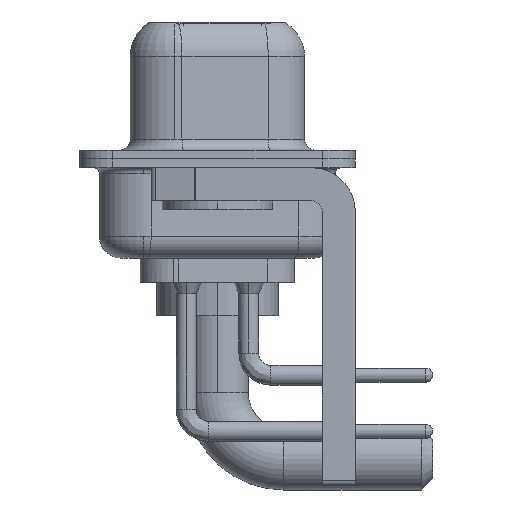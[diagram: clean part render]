
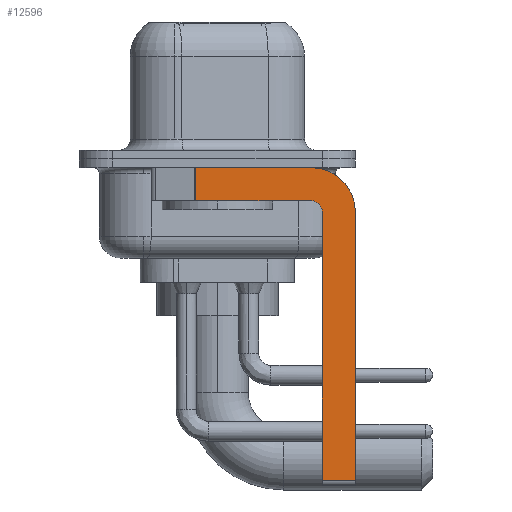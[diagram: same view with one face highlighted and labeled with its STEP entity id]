
A CAD part, left-side view. The second image highlights one B-rep face of the part: STEP entity #12596.
In plain terms, the highlighted planar face has unit normal (-1, 0, 0).
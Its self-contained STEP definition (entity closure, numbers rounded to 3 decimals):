
#85 = ORIENTED_EDGE ( 'NONE', *, *, #14228, .F. ) ;
#259 = LINE ( 'NONE', #1392, #5265 ) ;
#366 = VERTEX_POINT ( 'NONE', #14176 ) ;
#626 = DIRECTION ( 'NONE',  ( 0., 0., -1. ) ) ;
#1088 = LINE ( 'NONE', #5089, #1661 ) ;
#1392 = CARTESIAN_POINT ( 'NONE',  ( -2.9, -6.25, -2.4 ) ) ;
#1661 = VECTOR ( 'NONE', #9052, 1000. ) ;
#1817 = CARTESIAN_POINT ( 'NONE',  ( -2.9, 0.978, -1.9 ) ) ;
#1922 = FACE_OUTER_BOUND ( 'NONE', #5949, .T. ) ;
#2211 = VERTEX_POINT ( 'NONE', #9523 ) ;
#2514 = VECTOR ( 'NONE', #17074, 1000. ) ;
#2653 = VECTOR ( 'NONE', #3198, 1000. ) ;
#2788 = DIRECTION ( 'NONE',  ( 0., 0., -1. ) ) ;
#2790 = CIRCLE ( 'NONE', #15186, 0.5 ) ;
#3198 = DIRECTION ( 'NONE',  ( 0., 0., 1. ) ) ;
#3204 = CARTESIAN_POINT ( 'NONE',  ( -2.9, -4.25, -2.4 ) ) ;
#3291 = DIRECTION ( 'NONE',  ( 0., -1., 0. ) ) ;
#3436 = AXIS2_PLACEMENT_3D ( 'NONE', #14606, #17026, #2788 ) ;
#4014 = ORIENTED_EDGE ( 'NONE', *, *, #5808, .F. ) ;
#4592 = CARTESIAN_POINT ( 'NONE',  ( -2.9, 3., -0.4 ) ) ;
#4657 = VECTOR ( 'NONE', #3291, 1000. ) ;
#4873 = DIRECTION ( 'NONE',  ( 0., -1., 0. ) ) ;
#4947 = EDGE_CURVE ( 'NONE', #15247, #366, #14741, .T. ) ;
#5089 = CARTESIAN_POINT ( 'NONE',  ( -2.9, -4.25, -1.9 ) ) ;
#5265 = VECTOR ( 'NONE', #8153, 1000. ) ;
#5554 = ORIENTED_EDGE ( 'NONE', *, *, #7724, .F. ) ;
#5808 = EDGE_CURVE ( 'NONE', #10435, #2211, #11835, .T. ) ;
#5831 = VERTEX_POINT ( 'NONE', #13481 ) ;
#5949 = EDGE_LOOP ( 'NONE', ( #5554, #12577, #14090, #11803, #4014, #13817, #85, #15540 ) ) ;
#5972 = CARTESIAN_POINT ( 'NONE',  ( -2.9, -4.25, -2.4 ) ) ;
#6309 = AXIS2_PLACEMENT_3D ( 'NONE', #5972, #15040, #626 ) ;
#6530 = VERTEX_POINT ( 'NONE', #7363 ) ;
#7341 = CARTESIAN_POINT ( 'NONE',  ( -2.9, -4.75, -14.55 ) ) ;
#7363 = CARTESIAN_POINT ( 'NONE',  ( -2.9, 0.978, -0.4 ) ) ;
#7724 = EDGE_CURVE ( 'NONE', #6530, #15247, #16485, .T. ) ;
#8153 = DIRECTION ( 'NONE',  ( 0., 0., -1. ) ) ;
#8853 = VERTEX_POINT ( 'NONE', #12858 ) ;
#9012 = CARTESIAN_POINT ( 'NONE',  ( -2.9, -4.25, -14.55 ) ) ;
#9052 = DIRECTION ( 'NONE',  ( 0., 1., 0. ) ) ;
#9253 = CARTESIAN_POINT ( 'NONE',  ( -2.9, 0.978, -1.9 ) ) ;
#9269 = CARTESIAN_POINT ( 'NONE',  ( -2.9, -4.75, -14.8 ) ) ;
#9523 = CARTESIAN_POINT ( 'NONE',  ( -2.9, -4.75, -2.4 ) ) ;
#10075 = VERTEX_POINT ( 'NONE', #1817 ) ;
#10240 = VECTOR ( 'NONE', #4873, 1000. ) ;
#10435 = VERTEX_POINT ( 'NONE', #7341 ) ;
#10521 = CARTESIAN_POINT ( 'NONE',  ( -2.9, -4.25, -0.4 ) ) ;
#11152 = DIRECTION ( 'NONE',  ( -1., 0., 0. ) ) ;
#11803 = ORIENTED_EDGE ( 'NONE', *, *, #15772, .F. ) ;
#11835 = LINE ( 'NONE', #9269, #2653 ) ;
#12577 = ORIENTED_EDGE ( 'NONE', *, *, #14736, .T. ) ;
#12596 = ADVANCED_FACE ( 'NONE', ( #1922 ), #13759, .F. ) ;
#12858 = CARTESIAN_POINT ( 'NONE',  ( -2.9, -4.25, -1.9 ) ) ;
#13481 = CARTESIAN_POINT ( 'NONE',  ( -2.9, -6.25, -14.55 ) ) ;
#13759 = PLANE ( 'NONE',  #6309 ) ;
#13817 = ORIENTED_EDGE ( 'NONE', *, *, #14108, .T. ) ;
#14090 = ORIENTED_EDGE ( 'NONE', *, *, #15153, .F. ) ;
#14108 = EDGE_CURVE ( 'NONE', #10435, #5831, #15723, .T. ) ;
#14176 = CARTESIAN_POINT ( 'NONE',  ( -2.9, -6.25, -2.4 ) ) ;
#14228 = EDGE_CURVE ( 'NONE', #366, #5831, #259, .T. ) ;
#14411 = LINE ( 'NONE', #9253, #2514 ) ;
#14606 = CARTESIAN_POINT ( 'NONE',  ( -2.9, -4.25, -2.4 ) ) ;
#14736 = EDGE_CURVE ( 'NONE', #6530, #10075, #14411, .T. ) ;
#14741 = CIRCLE ( 'NONE', #3436, 2. ) ;
#15040 = DIRECTION ( 'NONE',  ( 1., 0., 0. ) ) ;
#15153 = EDGE_CURVE ( 'NONE', #8853, #10075, #1088, .T. ) ;
#15186 = AXIS2_PLACEMENT_3D ( 'NONE', #3204, #11152, #16404 ) ;
#15247 = VERTEX_POINT ( 'NONE', #10521 ) ;
#15540 = ORIENTED_EDGE ( 'NONE', *, *, #4947, .F. ) ;
#15723 = LINE ( 'NONE', #9012, #10240 ) ;
#15772 = EDGE_CURVE ( 'NONE', #2211, #8853, #2790, .T. ) ;
#16404 = DIRECTION ( 'NONE',  ( 0., 0., 1. ) ) ;
#16485 = LINE ( 'NONE', #4592, #4657 ) ;
#17026 = DIRECTION ( 'NONE',  ( 1., 0., 0. ) ) ;
#17074 = DIRECTION ( 'NONE',  ( 0., 0., -1. ) ) ;
